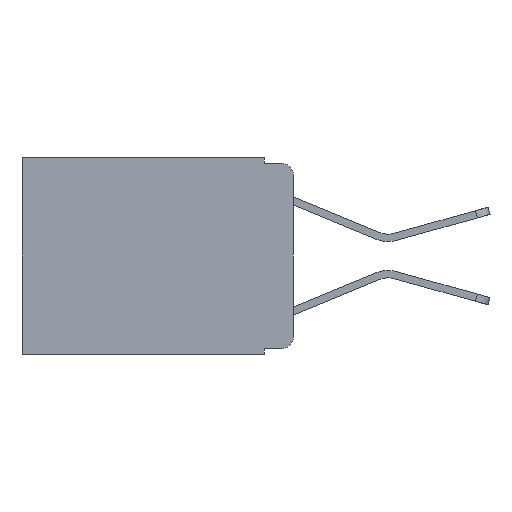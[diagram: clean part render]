
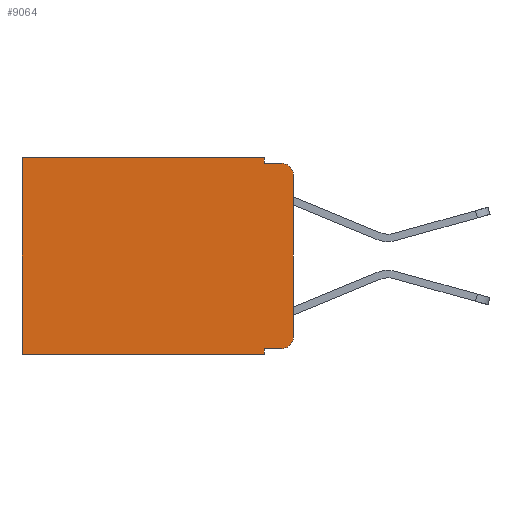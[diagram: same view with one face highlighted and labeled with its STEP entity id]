
A CAD part, left-side view. The second image highlights one B-rep face of the part: STEP entity #9064.
In plain terms, the highlighted planar face has unit normal (-1, 0, 0).
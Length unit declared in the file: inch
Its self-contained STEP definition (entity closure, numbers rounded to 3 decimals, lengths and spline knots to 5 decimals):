
#99 = EDGE_CURVE ( 'NONE', #5902, #6157, #10653, .T. ) ;
#347 = DIRECTION ( 'NONE',  ( 0., 0., -1. ) ) ;
#362 = DIRECTION ( 'NONE',  ( -1., 0., 0. ) ) ;
#384 = ORIENTED_EDGE ( 'NONE', *, *, #9022, .T. ) ;
#433 = DIRECTION ( 'NONE',  ( 0., -1., 0. ) ) ;
#792 = DIRECTION ( 'NONE',  ( 0., 0., -1. ) ) ;
#886 = CARTESIAN_POINT ( 'NONE',  ( 0.298, 0.051, -0.01 ) ) ;
#1027 = ORIENTED_EDGE ( 'NONE', *, *, #2419, .F. ) ;
#1229 = EDGE_CURVE ( 'NONE', #3460, #7861, #3218, .T. ) ;
#1297 = ORIENTED_EDGE ( 'NONE', *, *, #10072, .F. ) ;
#1317 = LINE ( 'NONE', #3613, #9836 ) ;
#1405 = VERTEX_POINT ( 'NONE', #7003 ) ;
#1624 = CARTESIAN_POINT ( 'NONE',  ( 0.298, 0., 0. ) ) ;
#1809 = DIRECTION ( 'NONE',  ( -1., 0., 0. ) ) ;
#1961 = ORIENTED_EDGE ( 'NONE', *, *, #99, .F. ) ;
#2210 = EDGE_CURVE ( 'NONE', #3672, #6642, #7184, .T. ) ;
#2411 = CARTESIAN_POINT ( 'NONE',  ( 0.298, 0.051, -0.333 ) ) ;
#2419 = EDGE_CURVE ( 'NONE', #3460, #5902, #8877, .T. ) ;
#2438 = DIRECTION ( 'NONE',  ( 0., -1., 0. ) ) ;
#2465 = DIRECTION ( 'NONE',  ( 0., 0., -1. ) ) ;
#2514 = VECTOR ( 'NONE', #2465, 39.37008 ) ;
#2687 = CIRCLE ( 'NONE', #6165, 0.02 ) ;
#2758 = DIRECTION ( 'NONE',  ( 0., 0., -1. ) ) ;
#2798 = CARTESIAN_POINT ( 'NONE',  ( 0.298, 0.051, -0.01 ) ) ;
#2805 = ORIENTED_EDGE ( 'NONE', *, *, #6995, .T. ) ;
#2811 = ORIENTED_EDGE ( 'NONE', *, *, #3365, .T. ) ;
#2857 = CARTESIAN_POINT ( 'NONE',  ( 0.298, 0.02, -0.333 ) ) ;
#3107 = CARTESIAN_POINT ( 'NONE',  ( 0.298, 0.473, -0.343 ) ) ;
#3208 = ORIENTED_EDGE ( 'NONE', *, *, #9144, .T. ) ;
#3218 = LINE ( 'NONE', #2411, #9936 ) ;
#3365 = EDGE_CURVE ( 'NONE', #6060, #6642, #3971, .T. ) ;
#3460 = VERTEX_POINT ( 'NONE', #6061 ) ;
#3599 = ORIENTED_EDGE ( 'NONE', *, *, #2210, .F. ) ;
#3610 = EDGE_LOOP ( 'NONE', ( #6114, #2811, #3599, #1297, #384, #2805, #1961, #1027, #6560, #3208 ) ) ;
#3613 = CARTESIAN_POINT ( 'NONE',  ( 0.298, 0., 0. ) ) ;
#3672 = VERTEX_POINT ( 'NONE', #2798 ) ;
#3859 = AXIS2_PLACEMENT_3D ( 'NONE', #10628, #6002, #792 ) ;
#3926 = LINE ( 'NONE', #8365, #5947 ) ;
#3971 = CIRCLE ( 'NONE', #7699, 0.02 ) ;
#4798 = CARTESIAN_POINT ( 'NONE',  ( 0.298, 0.02, -0.03 ) ) ;
#5131 = DIRECTION ( 'NONE',  ( 0., 0., -1. ) ) ;
#5152 = PLANE ( 'NONE',  #3859 ) ;
#5614 = LINE ( 'NONE', #8941, #9573 ) ;
#5690 = VERTEX_POINT ( 'NONE', #7079 ) ;
#5787 = DIRECTION ( 'NONE',  ( 0., 0., -1. ) ) ;
#5902 = VERTEX_POINT ( 'NONE', #6719 ) ;
#5947 = VECTOR ( 'NONE', #5131, 39.37008 ) ;
#6002 = DIRECTION ( 'NONE',  ( 1., 0., 0. ) ) ;
#6060 = VERTEX_POINT ( 'NONE', #7733 ) ;
#6061 = CARTESIAN_POINT ( 'NONE',  ( 0.298, 0.051, -0.333 ) ) ;
#6114 = ORIENTED_EDGE ( 'NONE', *, *, #8891, .F. ) ;
#6157 = VERTEX_POINT ( 'NONE', #3107 ) ;
#6165 = AXIS2_PLACEMENT_3D ( 'NONE', #6942, #1809, #7755 ) ;
#6312 = LINE ( 'NONE', #1624, #8674 ) ;
#6560 = ORIENTED_EDGE ( 'NONE', *, *, #1229, .T. ) ;
#6573 = VECTOR ( 'NONE', #10209, 39.37008 ) ;
#6642 = VERTEX_POINT ( 'NONE', #7156 ) ;
#6719 = CARTESIAN_POINT ( 'NONE',  ( 0.298, 0.051, -0.343 ) ) ;
#6942 = CARTESIAN_POINT ( 'NONE',  ( 0.298, 0.02, -0.313 ) ) ;
#6995 = EDGE_CURVE ( 'NONE', #10304, #6157, #3926, .T. ) ;
#7003 = CARTESIAN_POINT ( 'NONE',  ( 0.298, 0., -0.313 ) ) ;
#7079 = CARTESIAN_POINT ( 'NONE',  ( 0.298, 0.051, 0. ) ) ;
#7156 = CARTESIAN_POINT ( 'NONE',  ( 0.298, 0.02, -0.01 ) ) ;
#7184 = LINE ( 'NONE', #886, #10718 ) ;
#7578 = DIRECTION ( 'NONE',  ( 0., 1., 0. ) ) ;
#7699 = AXIS2_PLACEMENT_3D ( 'NONE', #4798, #362, #347 ) ;
#7733 = CARTESIAN_POINT ( 'NONE',  ( 0.298, 0., -0.03 ) ) ;
#7755 = DIRECTION ( 'NONE',  ( 0., 0., -1. ) ) ;
#7861 = VERTEX_POINT ( 'NONE', #2857 ) ;
#7957 = FACE_OUTER_BOUND ( 'NONE', #3610, .T. ) ;
#8365 = CARTESIAN_POINT ( 'NONE',  ( 0.298, 0.473, 0. ) ) ;
#8584 = CARTESIAN_POINT ( 'NONE',  ( 0.298, 0.051, 0. ) ) ;
#8653 = CARTESIAN_POINT ( 'NONE',  ( 0.298, 0., -0.343 ) ) ;
#8674 = VECTOR ( 'NONE', #7578, 39.37008 ) ;
#8877 = LINE ( 'NONE', #8584, #2514 ) ;
#8891 = EDGE_CURVE ( 'NONE', #6060, #1405, #1317, .T. ) ;
#8941 = CARTESIAN_POINT ( 'NONE',  ( 0.298, 0.051, 0. ) ) ;
#9022 = EDGE_CURVE ( 'NONE', #5690, #10304, #6312, .T. ) ;
#9064 = ADVANCED_FACE ( 'NONE', ( #7957 ), #5152, .F. ) ;
#9144 = EDGE_CURVE ( 'NONE', #7861, #1405, #2687, .T. ) ;
#9573 = VECTOR ( 'NONE', #5787, 39.37008 ) ;
#9836 = VECTOR ( 'NONE', #2758, 39.37008 ) ;
#9936 = VECTOR ( 'NONE', #2438, 39.37008 ) ;
#10072 = EDGE_CURVE ( 'NONE', #5690, #3672, #5614, .T. ) ;
#10209 = DIRECTION ( 'NONE',  ( 0., 1., 0. ) ) ;
#10304 = VERTEX_POINT ( 'NONE', #10726 ) ;
#10628 = CARTESIAN_POINT ( 'NONE',  ( 0.298, 0., 0. ) ) ;
#10653 = LINE ( 'NONE', #8653, #6573 ) ;
#10718 = VECTOR ( 'NONE', #433, 39.37008 ) ;
#10726 = CARTESIAN_POINT ( 'NONE',  ( 0.298, 0.473, 0. ) ) ;
